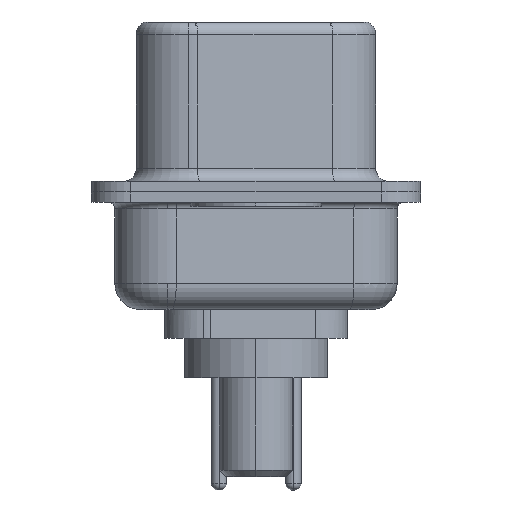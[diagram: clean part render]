
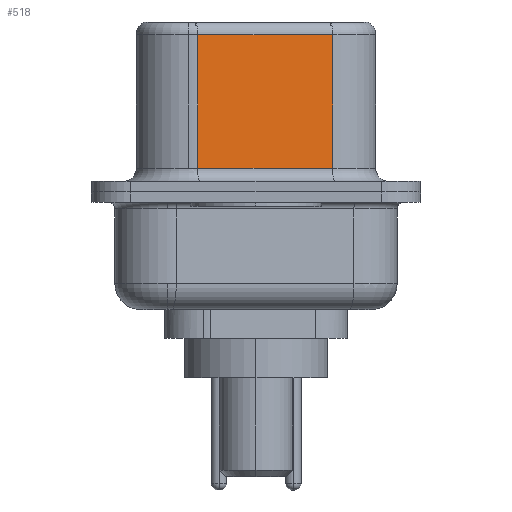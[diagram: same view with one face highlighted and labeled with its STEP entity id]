
A CAD part, left-side view. The second image highlights one B-rep face of the part: STEP entity #518.
In plain terms, the highlighted planar face has unit normal (-0.985, -0.174, 0).
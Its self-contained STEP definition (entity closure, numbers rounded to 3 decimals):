
#518 = ADVANCED_FACE ( 'NONE', ( #5784 ), #8859, .F. ) ;
#1519 = ORIENTED_EDGE ( 'NONE', *, *, #2343, .T. ) ;
#1795 = CARTESIAN_POINT ( 'NONE',  ( 3.67, 2.233, 0.9 ) ) ;
#2181 = CARTESIAN_POINT ( 'NONE',  ( 4.58, -2.927, 6.02 ) ) ;
#2343 = EDGE_CURVE ( 'NONE', #9963, #13305, #16392, .T. ) ;
#2694 = ORIENTED_EDGE ( 'NONE', *, *, #7015, .T. ) ;
#2701 = VERTEX_POINT ( 'NONE', #13129 ) ;
#2992 = LINE ( 'NONE', #18160, #11103 ) ;
#3606 = VERTEX_POINT ( 'NONE', #14503 ) ;
#4142 = LINE ( 'NONE', #2181, #15630 ) ;
#4486 = VECTOR ( 'NONE', #10107, 1000. ) ;
#4675 = VECTOR ( 'NONE', #5165, 1000. ) ;
#5165 = DIRECTION ( 'NONE',  ( 0., 0., -1. ) ) ;
#5255 = DIRECTION ( 'NONE',  ( -0.174, 0.985, 0. ) ) ;
#5784 = FACE_OUTER_BOUND ( 'NONE', #10248, .T. ) ;
#6829 = ORIENTED_EDGE ( 'NONE', *, *, #11582, .F. ) ;
#7015 = EDGE_CURVE ( 'NONE', #3606, #9963, #16562, .T. ) ;
#8859 = PLANE ( 'NONE',  #10608 ) ;
#9236 = DIRECTION ( 'NONE',  ( 0., 0., -1. ) ) ;
#9963 = VERTEX_POINT ( 'NONE', #1795 ) ;
#10107 = DIRECTION ( 'NONE',  ( 0.174, -0.985, 0. ) ) ;
#10248 = EDGE_LOOP ( 'NONE', ( #6829, #14128, #2694, #1519 ) ) ;
#10303 = CARTESIAN_POINT ( 'NONE',  ( 4.58, -2.927, 0.9 ) ) ;
#10608 = AXIS2_PLACEMENT_3D ( 'NONE', #11556, #17989, #5255 ) ;
#11103 = VECTOR ( 'NONE', #9236, 1000. ) ;
#11556 = CARTESIAN_POINT ( 'NONE',  ( 4.58, -2.927, 6.52 ) ) ;
#11582 = EDGE_CURVE ( 'NONE', #2701, #13305, #2992, .T. ) ;
#12747 = CARTESIAN_POINT ( 'NONE',  ( 3.67, 2.233, 6.52 ) ) ;
#12880 = DIRECTION ( 'NONE',  ( -0.174, 0.985, 0. ) ) ;
#13129 = CARTESIAN_POINT ( 'NONE',  ( 4.58, -2.927, 6.02 ) ) ;
#13305 = VERTEX_POINT ( 'NONE', #18580 ) ;
#14128 = ORIENTED_EDGE ( 'NONE', *, *, #17301, .T. ) ;
#14503 = CARTESIAN_POINT ( 'NONE',  ( 3.67, 2.233, 6.02 ) ) ;
#15630 = VECTOR ( 'NONE', #12880, 1000. ) ;
#16392 = LINE ( 'NONE', #10303, #4486 ) ;
#16562 = LINE ( 'NONE', #12747, #4675 ) ;
#17301 = EDGE_CURVE ( 'NONE', #2701, #3606, #4142, .T. ) ;
#17989 = DIRECTION ( 'NONE',  ( 0.985, 0.174, 0. ) ) ;
#18160 = CARTESIAN_POINT ( 'NONE',  ( 4.58, -2.927, 6.52 ) ) ;
#18580 = CARTESIAN_POINT ( 'NONE',  ( 4.58, -2.927, 0.9 ) ) ;
